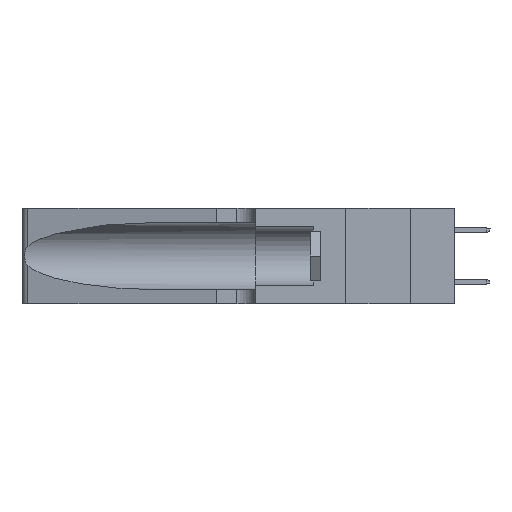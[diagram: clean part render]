
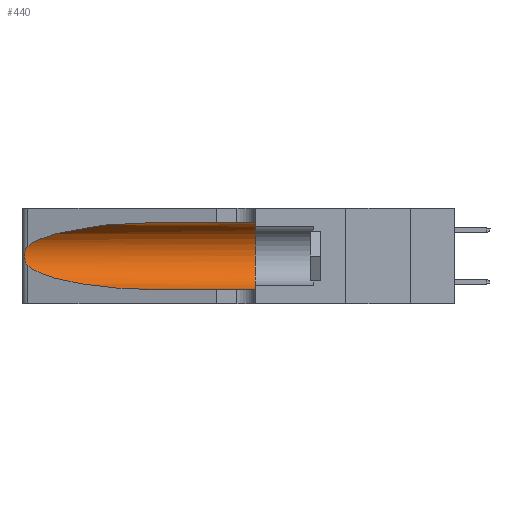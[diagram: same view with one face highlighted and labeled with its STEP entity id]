
A CAD part, left-side view. The second image highlights one B-rep face of the part: STEP entity #440.
In plain terms, the highlighted cylindrical face has radius 3.308 mm (diameter 6.617 mm), a partial arc.
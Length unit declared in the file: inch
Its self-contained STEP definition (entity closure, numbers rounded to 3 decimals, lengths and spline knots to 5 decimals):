
#440 = ADVANCED_FACE ( 'NONE', ( #21949 ), #12376, .F. ) ;
#1075 = CARTESIAN_POINT ( 'NONE',  ( 0.25787, 1.23484, 0.2124 ) ) ;
#1093 = ORIENTED_EDGE ( 'NONE', *, *, #23326, .T. ) ;
#1585 = EDGE_CURVE ( 'NONE', #16114, #16560, #1972, .T. ) ;
#1972 = LINE ( 'NONE', #7525, #3536 ) ;
#2240 = ORIENTED_EDGE ( 'NONE', *, *, #11881, .F. ) ;
#2481 =( BOUNDED_CURVE ( )  B_SPLINE_CURVE ( 3, ( #4340, #12048, #15920, #23630 ),
 .UNSPECIFIED., .F., .T. ) 
 B_SPLINE_CURVE_WITH_KNOTS ( ( 4, 4 ),
 ( 3.44316, 4.71239 ),
 .UNSPECIFIED. ) 
 CURVE ( )  GEOMETRIC_REPRESENTATION_ITEM ( )  RATIONAL_B_SPLINE_CURVE ( ( 1., 0.87, 0.87, 1. ) ) 
 REPRESENTATION_ITEM ( '' )  );
#2921 = VERTEX_POINT ( 'NONE', #14386 ) ;
#3192 = CARTESIAN_POINT ( 'NONE',  ( 0.1305, 0.35, 0.185 ) ) ;
#3277 = ORIENTED_EDGE ( 'NONE', *, *, #3291, .T. ) ;
#3291 = EDGE_CURVE ( 'NONE', #22132, #2921, #6795, .T. ) ;
#3434 =( BOUNDED_CURVE ( )  B_SPLINE_CURVE ( 3, ( #17370, #15462, #23173, #19262 ),
 .UNSPECIFIED., .F., .T. ) 
 B_SPLINE_CURVE_WITH_KNOTS ( ( 4, 4 ),
 ( 1.5708, 2.84003 ),
 .UNSPECIFIED. ) 
 CURVE ( )  GEOMETRIC_REPRESENTATION_ITEM ( )  RATIONAL_B_SPLINE_CURVE ( ( 1., 0.87, 0.87, 1. ) ) 
 REPRESENTATION_ITEM ( '' )  );
#3536 = VECTOR ( 'NONE', #15215, 39.37008 ) ;
#4340 = CARTESIAN_POINT ( 'NONE',  ( 0.25487, 1.22718, 0.14631 ) ) ;
#4875 = CARTESIAN_POINT ( 'NONE',  ( 0.26075, 1.23896, 0.19203 ) ) ;
#6764 = CARTESIAN_POINT ( 'NONE',  ( 0.25487, 1.22718, 0.14631 ) ) ;
#6795 = B_SPLINE_CURVE_WITH_KNOTS ( 'NONE', 3,
 ( #16328, #20255, #18607, #1075, #16458, #24163, #4875, #12577, #7003, #14701, #21908, #12696, #8901, #6764 ),
 .UNSPECIFIED., .F., .F.,
 ( 4, 2, 2, 2, 2, 2, 4 ),
 ( 0., 0.00027, 0.00053, 0.00107, 0.0016, 0.00187, 0.00214 ),
 .UNSPECIFIED. ) ;
#7003 = CARTESIAN_POINT ( 'NONE',  ( 0.26017, 1.23833, 0.17102 ) ) ;
#7321 = CARTESIAN_POINT ( 'NONE',  ( 0.25487, 1.22718, 0.22369 ) ) ;
#7452 = EDGE_CURVE ( 'NONE', #16114, #22132, #3434, .T. ) ;
#7525 = CARTESIAN_POINT ( 'NONE',  ( 0.1305, 1.61858, 0.31525 ) ) ;
#7708 = LINE ( 'NONE', #20683, #22583 ) ;
#8901 = CARTESIAN_POINT ( 'NONE',  ( 0.25555, 1.22993, 0.14849 ) ) ;
#9568 = VERTEX_POINT ( 'NONE', #20604 ) ;
#10134 = ORIENTED_EDGE ( 'NONE', *, *, #1585, .F. ) ;
#10602 = CIRCLE ( 'NONE', #24707, 0.13025 ) ;
#11155 = VERTEX_POINT ( 'NONE', #13577 ) ;
#11837 = EDGE_CURVE ( 'NONE', #2921, #9568, #2481, .T. ) ;
#11881 = EDGE_CURVE ( 'NONE', #16560, #11155, #10602, .T. ) ;
#12048 = CARTESIAN_POINT ( 'NONE',  ( 0.2373, 1.15595, 0.08982 ) ) ;
#12376 = CYLINDRICAL_SURFACE ( 'NONE', #21207, 0.13025 ) ;
#12577 = CARTESIAN_POINT ( 'NONE',  ( 0.26075, 1.23896, 0.178 ) ) ;
#12696 = CARTESIAN_POINT ( 'NONE',  ( 0.25639, 1.23186, 0.15144 ) ) ;
#13577 = CARTESIAN_POINT ( 'NONE',  ( 0.1305, 0.35, 0.05475 ) ) ;
#13975 = CARTESIAN_POINT ( 'NONE',  ( 0.1305, 0.72297, 0.31525 ) ) ;
#14370 = CARTESIAN_POINT ( 'NONE',  ( 0.1305, 1.61858, 0.185 ) ) ;
#14386 = CARTESIAN_POINT ( 'NONE',  ( 0.25487, 1.22718, 0.14631 ) ) ;
#14409 = DIRECTION ( 'NONE',  ( 0., 1., 0. ) ) ;
#14701 = CARTESIAN_POINT ( 'NONE',  ( 0.25856, 1.23593, 0.16098 ) ) ;
#14916 = DIRECTION ( 'NONE',  ( 0., 0., 1. ) ) ;
#15215 = DIRECTION ( 'NONE',  ( 0., -1., 0. ) ) ;
#15462 = CARTESIAN_POINT ( 'NONE',  ( 0.18966, 0.96281, 0.31525 ) ) ;
#15920 = CARTESIAN_POINT ( 'NONE',  ( 0.18966, 0.96281, 0.05475 ) ) ;
#15945 = CARTESIAN_POINT ( 'NONE',  ( 0.1305, 0.35, 0.31525 ) ) ;
#16114 = VERTEX_POINT ( 'NONE', #13975 ) ;
#16328 = CARTESIAN_POINT ( 'NONE',  ( 0.25487, 1.22718, 0.22369 ) ) ;
#16458 = CARTESIAN_POINT ( 'NONE',  ( 0.25854, 1.2359, 0.20912 ) ) ;
#16560 = VERTEX_POINT ( 'NONE', #15945 ) ;
#17121 = DIRECTION ( 'NONE',  ( 0., -1., 0. ) ) ;
#17370 = CARTESIAN_POINT ( 'NONE',  ( 0.1305, 0.72297, 0.31525 ) ) ;
#18607 = CARTESIAN_POINT ( 'NONE',  ( 0.25639, 1.23184, 0.21858 ) ) ;
#19262 = CARTESIAN_POINT ( 'NONE',  ( 0.25487, 1.22718, 0.22369 ) ) ;
#20255 = CARTESIAN_POINT ( 'NONE',  ( 0.25555, 1.22994, 0.2215 ) ) ;
#20604 = CARTESIAN_POINT ( 'NONE',  ( 0.1305, 0.72297, 0.05475 ) ) ;
#20683 = CARTESIAN_POINT ( 'NONE',  ( 0.1305, 1.61858, 0.05475 ) ) ;
#20820 = DIRECTION ( 'NONE',  ( 0., -1., 0. ) ) ;
#21207 = AXIS2_PLACEMENT_3D ( 'NONE', #14370, #17121, #22821 ) ;
#21579 = EDGE_LOOP ( 'NONE', ( #22252, #3277, #24810, #1093, #2240, #10134 ) ) ;
#21908 = CARTESIAN_POINT ( 'NONE',  ( 0.25789, 1.23486, 0.15765 ) ) ;
#21949 = FACE_OUTER_BOUND ( 'NONE', #21579, .T. ) ;
#22132 = VERTEX_POINT ( 'NONE', #7321 ) ;
#22252 = ORIENTED_EDGE ( 'NONE', *, *, #7452, .T. ) ;
#22583 = VECTOR ( 'NONE', #20820, 39.37008 ) ;
#22821 = DIRECTION ( 'NONE',  ( 0., 0., -1. ) ) ;
#23173 = CARTESIAN_POINT ( 'NONE',  ( 0.2373, 1.15595, 0.28018 ) ) ;
#23326 = EDGE_CURVE ( 'NONE', #9568, #11155, #7708, .T. ) ;
#23630 = CARTESIAN_POINT ( 'NONE',  ( 0.1305, 0.72297, 0.05475 ) ) ;
#24163 = CARTESIAN_POINT ( 'NONE',  ( 0.26018, 1.23835, 0.19895 ) ) ;
#24707 = AXIS2_PLACEMENT_3D ( 'NONE', #3192, #14409, #14916 ) ;
#24810 = ORIENTED_EDGE ( 'NONE', *, *, #11837, .T. ) ;
